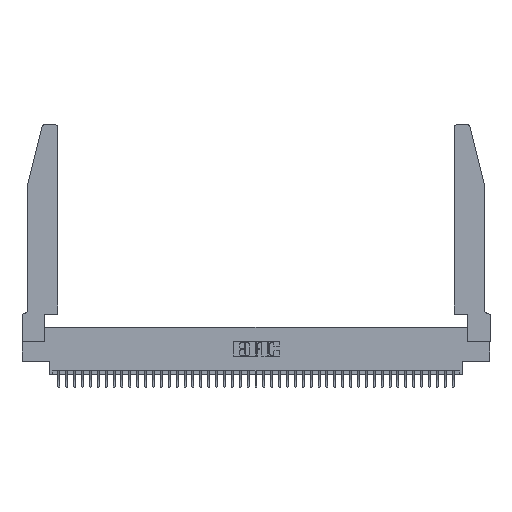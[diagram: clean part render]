
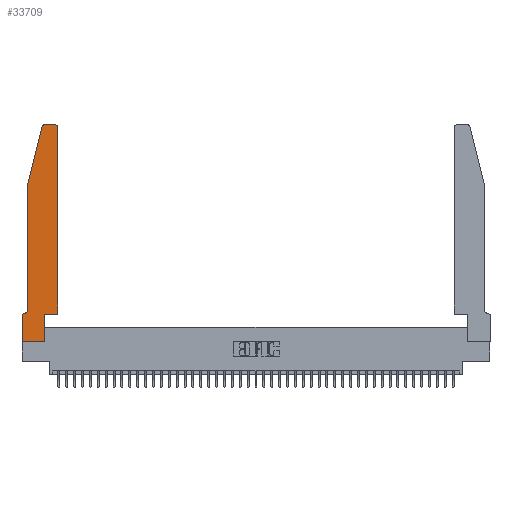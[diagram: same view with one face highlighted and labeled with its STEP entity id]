
A CAD part, top view. The second image highlights one B-rep face of the part: STEP entity #33709.
In plain terms, the highlighted planar face has unit normal (0, 0, 1).
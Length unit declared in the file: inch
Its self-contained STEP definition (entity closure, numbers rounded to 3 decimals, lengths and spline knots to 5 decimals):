
#260 = VERTEX_POINT ( 'NONE', #6517 ) ;
#1629 = EDGE_CURVE ( 'NONE', #3356, #260, #36575, .T. ) ;
#2278 = LINE ( 'NONE', #13235, #11512 ) ;
#2984 = DIRECTION ( 'NONE',  ( 1., 0., 0. ) ) ;
#3164 = CARTESIAN_POINT ( 'NONE',  ( 0.0055, 0.42, 0.37 ) ) ;
#3356 = VERTEX_POINT ( 'NONE', #31225 ) ;
#3388 = EDGE_CURVE ( 'NONE', #30642, #39408, #31816, .T. ) ;
#3767 = VERTEX_POINT ( 'NONE', #10203 ) ;
#4224 = DIRECTION ( 'NONE',  ( -0.239, -0.971, 0. ) ) ;
#4319 = CARTESIAN_POINT ( 'NONE',  ( 0.4505, 0.35, 0.37 ) ) ;
#4556 = VERTEX_POINT ( 'NONE', #26040 ) ;
#5630 = CIRCLE ( 'NONE', #31453, 0.07 ) ;
#5992 = ORIENTED_EDGE ( 'NONE', *, *, #38533, .T. ) ;
#6234 = VECTOR ( 'NONE', #43447, 39.37008 ) ;
#6517 = CARTESIAN_POINT ( 'NONE',  ( 0.0755, 0.42, 0.37 ) ) ;
#6637 = CARTESIAN_POINT ( 'NONE',  ( 0., 0., 0.37 ) ) ;
#6688 = DIRECTION ( 'NONE',  ( -1., 0., 0. ) ) ;
#6880 = EDGE_CURVE ( 'NONE', #29753, #3356, #8835, .T. ) ;
#7105 = LINE ( 'NONE', #32154, #31990 ) ;
#7918 = DIRECTION ( 'NONE',  ( 0., 1., 0. ) ) ;
#8126 = CARTESIAN_POINT ( 'NONE',  ( 0., 0., 0.37 ) ) ;
#8835 = LINE ( 'NONE', #34625, #24790 ) ;
#9082 = VERTEX_POINT ( 'NONE', #30730 ) ;
#10203 = CARTESIAN_POINT ( 'NONE',  ( 0.4505, 2.72, 0.37 ) ) ;
#10924 = CARTESIAN_POINT ( 'NONE',  ( 0., 0., 0.37 ) ) ;
#11512 = VECTOR ( 'NONE', #30054, 39.37008 ) ;
#13235 = CARTESIAN_POINT ( 'NONE',  ( 0.2865, 0.35, 0.37 ) ) ;
#13510 = VERTEX_POINT ( 'NONE', #4319 ) ;
#14479 = CARTESIAN_POINT ( 'NONE',  ( 0.2865, 0., 0.37 ) ) ;
#15407 = DIRECTION ( 'NONE',  ( 1., 0., 0. ) ) ;
#15650 = CARTESIAN_POINT ( 'NONE',  ( 0.4205, 2.75, 0.37 ) ) ;
#16224 = DIRECTION ( 'NONE',  ( 0., -1., 0. ) ) ;
#16822 = CARTESIAN_POINT ( 'NONE',  ( 0., 0.35, 0.37 ) ) ;
#17428 = DIRECTION ( 'NONE',  ( 0., 0., 1. ) ) ;
#17694 = ORIENTED_EDGE ( 'NONE', *, *, #22931, .T. ) ;
#18662 = ORIENTED_EDGE ( 'NONE', *, *, #31776, .T. ) ;
#18684 = VERTEX_POINT ( 'NONE', #41757 ) ;
#19069 = ORIENTED_EDGE ( 'NONE', *, *, #42303, .T. ) ;
#20046 = CARTESIAN_POINT ( 'NONE',  ( 0.0755, 0.35, 0.37 ) ) ;
#20230 = DIRECTION ( 'NONE',  ( 0., 0., 1. ) ) ;
#20283 = ORIENTED_EDGE ( 'NONE', *, *, #36328, .T. ) ;
#21655 = CARTESIAN_POINT ( 'NONE',  ( 0.4505, 0.35, 0.37 ) ) ;
#21706 = ORIENTED_EDGE ( 'NONE', *, *, #6880, .T. ) ;
#22931 = EDGE_CURVE ( 'NONE', #13510, #3767, #25934, .T. ) ;
#22939 = VECTOR ( 'NONE', #31790, 39.37008 ) ;
#23513 = DIRECTION ( 'NONE',  ( 0., 0., 1. ) ) ;
#23988 = EDGE_CURVE ( 'NONE', #39408, #39557, #2278, .T. ) ;
#24573 = DIRECTION ( 'NONE',  ( 0., -1., 0. ) ) ;
#24790 = VECTOR ( 'NONE', #4224, 39.37008 ) ;
#24875 = VECTOR ( 'NONE', #7918, 39.37008 ) ;
#24911 = CARTESIAN_POINT ( 'NONE',  ( 0.2605, 2.75, 0.37 ) ) ;
#24983 = EDGE_CURVE ( 'NONE', #39557, #13510, #7105, .T. ) ;
#25146 = ORIENTED_EDGE ( 'NONE', *, *, #24983, .T. ) ;
#25398 = LINE ( 'NONE', #20046, #6234 ) ;
#25895 = CARTESIAN_POINT ( 'NONE',  ( 0.25487, 2.72718, 0.37 ) ) ;
#25934 = LINE ( 'NONE', #21655, #24875 ) ;
#25954 = AXIS2_PLACEMENT_3D ( 'NONE', #37490, #17428, #40860 ) ;
#26040 = CARTESIAN_POINT ( 'NONE',  ( 0.0055, 0.35, 0.37 ) ) ;
#26894 = FACE_OUTER_BOUND ( 'NONE', #31739, .T. ) ;
#26931 = ORIENTED_EDGE ( 'NONE', *, *, #33079, .T. ) ;
#27058 = DIRECTION ( 'NONE',  ( 0., 0., -1. ) ) ;
#27560 = ORIENTED_EDGE ( 'NONE', *, *, #23988, .T. ) ;
#28604 = CARTESIAN_POINT ( 'NONE',  ( 0.2865, 0.35, 0.37 ) ) ;
#28709 = VECTOR ( 'NONE', #16224, 39.37008 ) ;
#29572 = CIRCLE ( 'NONE', #25954, 0.03 ) ;
#29753 = VERTEX_POINT ( 'NONE', #25895 ) ;
#30054 = DIRECTION ( 'NONE',  ( 0., 1., 0. ) ) ;
#30165 = AXIS2_PLACEMENT_3D ( 'NONE', #43530, #23513, #2984 ) ;
#30642 = VERTEX_POINT ( 'NONE', #6637 ) ;
#30730 = CARTESIAN_POINT ( 'NONE',  ( 0., 0.35, 0.37 ) ) ;
#31225 = CARTESIAN_POINT ( 'NONE',  ( 0.0755, 2., 0.37 ) ) ;
#31453 = AXIS2_PLACEMENT_3D ( 'NONE', #3164, #27058, #6688 ) ;
#31739 = EDGE_LOOP ( 'NONE', ( #20283, #18662, #21706, #43094, #41387, #5992, #19069, #34904, #27560, #25146, #17694, #26931 ) ) ;
#31776 = EDGE_CURVE ( 'NONE', #18684, #29753, #29572, .T. ) ;
#31790 = DIRECTION ( 'NONE',  ( 1., 0., 0. ) ) ;
#31816 = LINE ( 'NONE', #8126, #22939 ) ;
#31990 = VECTOR ( 'NONE', #15407, 39.37008 ) ;
#32154 = CARTESIAN_POINT ( 'NONE',  ( 0.4505, 0.35, 0.37 ) ) ;
#33079 = EDGE_CURVE ( 'NONE', #3767, #35899, #34270, .T. ) ;
#33709 = ADVANCED_FACE ( 'NONE', ( #26894 ), #36897, .T. ) ;
#34270 = CIRCLE ( 'NONE', #30165, 0.03 ) ;
#34401 = VECTOR ( 'NONE', #24573, 39.37008 ) ;
#34625 = CARTESIAN_POINT ( 'NONE',  ( 0.0755, 2., 0.37 ) ) ;
#34904 = ORIENTED_EDGE ( 'NONE', *, *, #3388, .T. ) ;
#35224 = AXIS2_PLACEMENT_3D ( 'NONE', #16822, #20230, #43626 ) ;
#35899 = VERTEX_POINT ( 'NONE', #15650 ) ;
#36318 = CARTESIAN_POINT ( 'NONE',  ( 0.0755, 2., 0.37 ) ) ;
#36328 = EDGE_CURVE ( 'NONE', #35899, #18684, #39197, .T. ) ;
#36500 = LINE ( 'NONE', #10924, #34401 ) ;
#36575 = LINE ( 'NONE', #36318, #28709 ) ;
#36897 = PLANE ( 'NONE',  #35224 ) ;
#37490 = CARTESIAN_POINT ( 'NONE',  ( 0.284, 2.72, 0.37 ) ) ;
#38131 = VECTOR ( 'NONE', #38339, 39.37008 ) ;
#38339 = DIRECTION ( 'NONE',  ( -1., 0., 0. ) ) ;
#38533 = EDGE_CURVE ( 'NONE', #4556, #9082, #25398, .T. ) ;
#39161 = EDGE_CURVE ( 'NONE', #260, #4556, #5630, .T. ) ;
#39197 = LINE ( 'NONE', #24911, #38131 ) ;
#39408 = VERTEX_POINT ( 'NONE', #14479 ) ;
#39557 = VERTEX_POINT ( 'NONE', #28604 ) ;
#40860 = DIRECTION ( 'NONE',  ( 1., 0., 0. ) ) ;
#41387 = ORIENTED_EDGE ( 'NONE', *, *, #39161, .T. ) ;
#41757 = CARTESIAN_POINT ( 'NONE',  ( 0.284, 2.75, 0.37 ) ) ;
#42303 = EDGE_CURVE ( 'NONE', #9082, #30642, #36500, .T. ) ;
#43094 = ORIENTED_EDGE ( 'NONE', *, *, #1629, .T. ) ;
#43447 = DIRECTION ( 'NONE',  ( -1., 0., 0. ) ) ;
#43530 = CARTESIAN_POINT ( 'NONE',  ( 0.4205, 2.72, 0.37 ) ) ;
#43626 = DIRECTION ( 'NONE',  ( 1., 0., 0. ) ) ;
